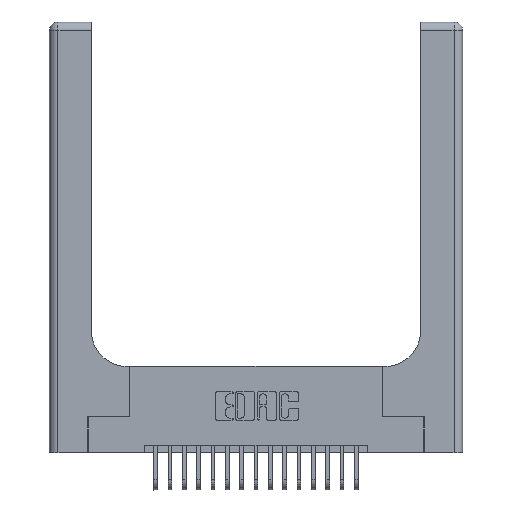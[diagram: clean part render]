
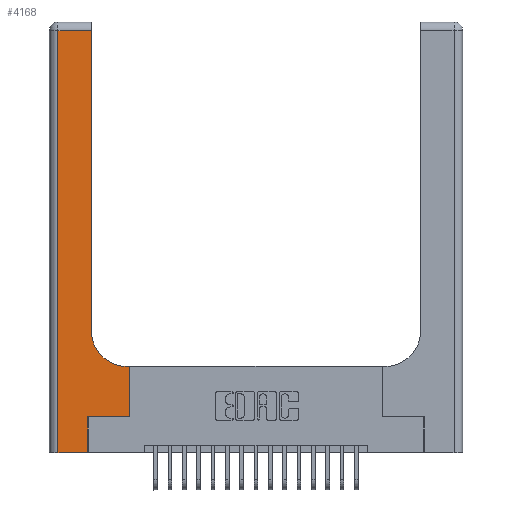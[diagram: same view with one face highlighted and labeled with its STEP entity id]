
A CAD part, top view. The second image highlights one B-rep face of the part: STEP entity #4168.
In plain terms, the highlighted planar face has unit normal (0, 0, 1).
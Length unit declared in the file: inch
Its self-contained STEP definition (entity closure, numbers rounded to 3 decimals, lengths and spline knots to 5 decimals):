
#257 = VECTOR ( 'NONE', #4914, 39.37008 ) ;
#376 = EDGE_LOOP ( 'NONE', ( #16676, #6695, #11344, #4456, #5944, #11097, #15723, #5231, #5710 ) ) ;
#1040 = VERTEX_POINT ( 'NONE', #7124 ) ;
#1232 = CARTESIAN_POINT ( 'NONE',  ( 0., 0., 0.37 ) ) ;
#1435 = VECTOR ( 'NONE', #20124, 39.37008 ) ;
#1521 = CARTESIAN_POINT ( 'NONE',  ( 0.5415, 0.85, 0.37 ) ) ;
#1550 = PLANE ( 'NONE',  #12155 ) ;
#1559 = EDGE_CURVE ( 'NONE', #9643, #18114, #16382, .T. ) ;
#1802 = VECTOR ( 'NONE', #18636, 39.37008 ) ;
#1975 = LINE ( 'NONE', #14467, #5637 ) ;
#2376 = VECTOR ( 'NONE', #10588, 39.37008 ) ;
#2454 = VECTOR ( 'NONE', #15893, 39.37008 ) ;
#3091 = DIRECTION ( 'NONE',  ( 1., 0., 0. ) ) ;
#3116 = EDGE_CURVE ( 'NONE', #6466, #9643, #18994, .T. ) ;
#4168 = ADVANCED_FACE ( 'NONE', ( #15050 ), #1550, .F. ) ;
#4456 = ORIENTED_EDGE ( 'NONE', *, *, #12256, .T. ) ;
#4590 = CARTESIAN_POINT ( 'NONE',  ( 0.269, 0.25, 0.37 ) ) ;
#4663 = DIRECTION ( 'NONE',  ( -1., 0., 0. ) ) ;
#4796 = DIRECTION ( 'NONE',  ( 0., 1., 0. ) ) ;
#4813 = CARTESIAN_POINT ( 'NONE',  ( 0.2915, 0.85, 0.37 ) ) ;
#4844 = EDGE_CURVE ( 'NONE', #7478, #5960, #8262, .T. ) ;
#4914 = DIRECTION ( 'NONE',  ( 0., 1., 0. ) ) ;
#5231 = ORIENTED_EDGE ( 'NONE', *, *, #15661, .T. ) ;
#5426 = VECTOR ( 'NONE', #11090, 39.37008 ) ;
#5637 = VECTOR ( 'NONE', #9826, 39.37008 ) ;
#5710 = ORIENTED_EDGE ( 'NONE', *, *, #4844, .T. ) ;
#5944 = ORIENTED_EDGE ( 'NONE', *, *, #15105, .T. ) ;
#5960 = VERTEX_POINT ( 'NONE', #4813 ) ;
#6466 = VERTEX_POINT ( 'NONE', #16758 ) ;
#6589 = EDGE_CURVE ( 'NONE', #16001, #1040, #10116, .T. ) ;
#6695 = ORIENTED_EDGE ( 'NONE', *, *, #6589, .T. ) ;
#7124 = CARTESIAN_POINT ( 'NONE',  ( 0.06, 2.94, 0.37 ) ) ;
#7478 = VERTEX_POINT ( 'NONE', #20000 ) ;
#8262 = CIRCLE ( 'NONE', #10302, 0.25 ) ;
#8393 = CARTESIAN_POINT ( 'NONE',  ( 0.5585, 0.6, 0.37 ) ) ;
#8622 = VERTEX_POINT ( 'NONE', #10672 ) ;
#9587 = LINE ( 'NONE', #14144, #5426 ) ;
#9643 = VERTEX_POINT ( 'NONE', #14650 ) ;
#9826 = DIRECTION ( 'NONE',  ( 0., -1., 0. ) ) ;
#10116 = LINE ( 'NONE', #12411, #1802 ) ;
#10302 = AXIS2_PLACEMENT_3D ( 'NONE', #1521, #12470, #3091 ) ;
#10384 = CARTESIAN_POINT ( 'NONE',  ( 0.2915, 2.94, 0.37 ) ) ;
#10588 = DIRECTION ( 'NONE',  ( 1., 0., 0. ) ) ;
#10672 = CARTESIAN_POINT ( 'NONE',  ( 0.06, 0., 0.37 ) ) ;
#10944 = VERTEX_POINT ( 'NONE', #19531 ) ;
#11089 = VECTOR ( 'NONE', #4796, 39.37008 ) ;
#11090 = DIRECTION ( 'NONE',  ( -1., 0., 0. ) ) ;
#11097 = ORIENTED_EDGE ( 'NONE', *, *, #3116, .T. ) ;
#11344 = ORIENTED_EDGE ( 'NONE', *, *, #16375, .T. ) ;
#12155 = AXIS2_PLACEMENT_3D ( 'NONE', #12493, #14039, #4663 ) ;
#12256 = EDGE_CURVE ( 'NONE', #8622, #10944, #14847, .T. ) ;
#12411 = CARTESIAN_POINT ( 'NONE',  ( 0., 2.94, 0.37 ) ) ;
#12470 = DIRECTION ( 'NONE',  ( 0., 0., -1. ) ) ;
#12493 = CARTESIAN_POINT ( 'NONE',  ( 0., 3., 0.37 ) ) ;
#14039 = DIRECTION ( 'NONE',  ( 0., 0., -1. ) ) ;
#14144 = CARTESIAN_POINT ( 'NONE',  ( 0.2915, 0.6, 0.37 ) ) ;
#14292 = CARTESIAN_POINT ( 'NONE',  ( 0.5585, 0.25, 0.37 ) ) ;
#14401 = CARTESIAN_POINT ( 'NONE',  ( 0.2915, 3., 0.37 ) ) ;
#14467 = CARTESIAN_POINT ( 'NONE',  ( 0.06, 3., 0.37 ) ) ;
#14650 = CARTESIAN_POINT ( 'NONE',  ( 0.5585, 0.25, 0.37 ) ) ;
#14847 = LINE ( 'NONE', #1232, #2376 ) ;
#15050 = FACE_OUTER_BOUND ( 'NONE', #376, .T. ) ;
#15105 = EDGE_CURVE ( 'NONE', #10944, #6466, #19347, .T. ) ;
#15422 = LINE ( 'NONE', #14401, #2454 ) ;
#15661 = EDGE_CURVE ( 'NONE', #18114, #7478, #9587, .T. ) ;
#15723 = ORIENTED_EDGE ( 'NONE', *, *, #1559, .T. ) ;
#15736 = CARTESIAN_POINT ( 'NONE',  ( 0.269, 0., 0.37 ) ) ;
#15893 = DIRECTION ( 'NONE',  ( 0., 1., 0. ) ) ;
#16001 = VERTEX_POINT ( 'NONE', #10384 ) ;
#16326 = EDGE_CURVE ( 'NONE', #5960, #16001, #15422, .T. ) ;
#16375 = EDGE_CURVE ( 'NONE', #1040, #8622, #1975, .T. ) ;
#16382 = LINE ( 'NONE', #14292, #257 ) ;
#16676 = ORIENTED_EDGE ( 'NONE', *, *, #16326, .T. ) ;
#16758 = CARTESIAN_POINT ( 'NONE',  ( 0.269, 0.25, 0.37 ) ) ;
#18114 = VERTEX_POINT ( 'NONE', #8393 ) ;
#18636 = DIRECTION ( 'NONE',  ( -1., 0., 0. ) ) ;
#18994 = LINE ( 'NONE', #4590, #1435 ) ;
#19347 = LINE ( 'NONE', #15736, #11089 ) ;
#19531 = CARTESIAN_POINT ( 'NONE',  ( 0.269, 0., 0.37 ) ) ;
#20000 = CARTESIAN_POINT ( 'NONE',  ( 0.5415, 0.6, 0.37 ) ) ;
#20124 = DIRECTION ( 'NONE',  ( 1., 0., 0. ) ) ;
